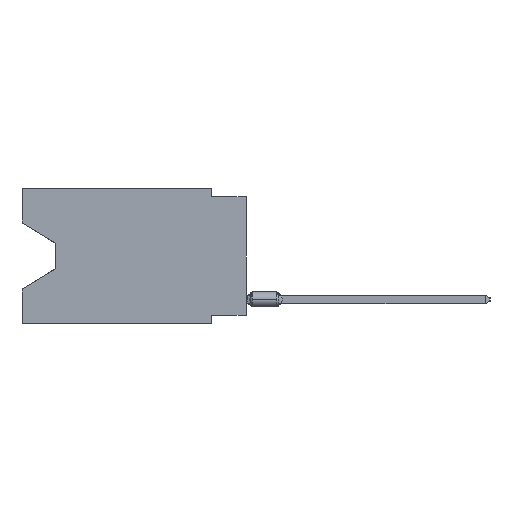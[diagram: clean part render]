
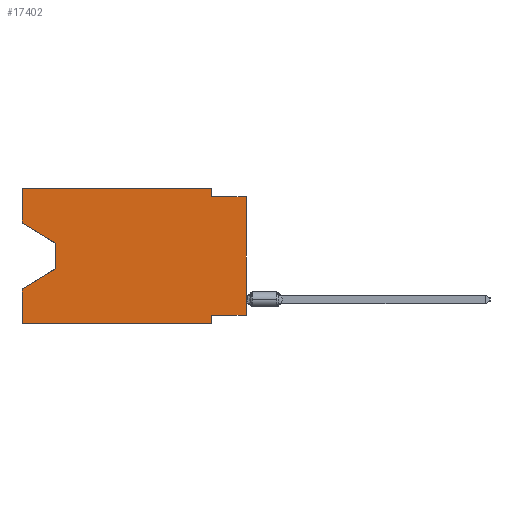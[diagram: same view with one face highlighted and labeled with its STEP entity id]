
A CAD part, left-side view. The second image highlights one B-rep face of the part: STEP entity #17402.
In plain terms, the highlighted planar face has unit normal (-1, 0, 0).
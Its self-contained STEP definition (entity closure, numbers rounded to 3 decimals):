
#490 = ORIENTED_EDGE ( 'NONE', *, *, #6611, .F. ) ;
#867 = EDGE_CURVE ( 'NONE', #46629, #14320, #31707, .T. ) ;
#884 = LINE ( 'NONE', #30411, #24680 ) ;
#920 = EDGE_CURVE ( 'NONE', #15908, #10579, #16933, .T. ) ;
#1246 = LINE ( 'NONE', #15779, #7198 ) ;
#1443 = PLANE ( 'NONE',  #12343 ) ;
#2384 = VECTOR ( 'NONE', #34736, 1000. ) ;
#2610 = ORIENTED_EDGE ( 'NONE', *, *, #28132, .T. ) ;
#2934 = VERTEX_POINT ( 'NONE', #3362 ) ;
#3362 = CARTESIAN_POINT ( 'NONE',  ( 0., 13.97, -5.893 ) ) ;
#3417 = VERTEX_POINT ( 'NONE', #43603 ) ;
#4393 = VERTEX_POINT ( 'NONE', #26133 ) ;
#4486 = VERTEX_POINT ( 'NONE', #42276 ) ;
#5261 = DIRECTION ( 'NONE',  ( 0., -1., 0. ) ) ;
#6031 = CARTESIAN_POINT ( 'NONE',  ( 0., 13.97, -5.893 ) ) ;
#6139 = CARTESIAN_POINT ( 'NONE',  ( 0., 16.383, 0. ) ) ;
#6611 = EDGE_CURVE ( 'NONE', #37154, #45701, #17321, .T. ) ;
#6680 = VECTOR ( 'NONE', #11840, 1000. ) ;
#6892 = ORIENTED_EDGE ( 'NONE', *, *, #28656, .F. ) ;
#7198 = VECTOR ( 'NONE', #44785, 1000. ) ;
#7208 = ORIENTED_EDGE ( 'NONE', *, *, #8430, .T. ) ;
#8305 = CARTESIAN_POINT ( 'NONE',  ( 0., 16.383, -9.906 ) ) ;
#8385 = ORIENTED_EDGE ( 'NONE', *, *, #867, .T. ) ;
#8430 = EDGE_CURVE ( 'NONE', #14320, #2934, #13546, .T. ) ;
#9372 = EDGE_CURVE ( 'NONE', #3417, #26324, #43079, .T. ) ;
#10579 = VERTEX_POINT ( 'NONE', #18112 ) ;
#10621 = VECTOR ( 'NONE', #16477, 1000. ) ;
#11178 = DIRECTION ( 'NONE',  ( 0., -1., 0. ) ) ;
#11235 = EDGE_CURVE ( 'NONE', #26324, #4393, #38291, .T. ) ;
#11840 = DIRECTION ( 'NONE',  ( 0., 0., -1. ) ) ;
#12310 = DIRECTION ( 'NONE',  ( 0., 0., 1. ) ) ;
#12343 = AXIS2_PLACEMENT_3D ( 'NONE', #15499, #12640, #41662 ) ;
#12640 = DIRECTION ( 'NONE',  ( 1., 0., 0. ) ) ;
#12672 = CARTESIAN_POINT ( 'NONE',  ( 0., 16.383, 0. ) ) ;
#12894 = VECTOR ( 'NONE', #20752, 1000. ) ;
#13381 = CARTESIAN_POINT ( 'NONE',  ( 0., 0., -0.635 ) ) ;
#13546 = LINE ( 'NONE', #28068, #6680 ) ;
#14320 = VERTEX_POINT ( 'NONE', #46619 ) ;
#15499 = CARTESIAN_POINT ( 'NONE',  ( 0., 16.383, 0. ) ) ;
#15779 = CARTESIAN_POINT ( 'NONE',  ( 0., 2.54, 0. ) ) ;
#15908 = VERTEX_POINT ( 'NONE', #35301 ) ;
#16450 = VECTOR ( 'NONE', #11178, 1000. ) ;
#16477 = DIRECTION ( 'NONE',  ( 0., 0., 1. ) ) ;
#16847 = ORIENTED_EDGE ( 'NONE', *, *, #9372, .F. ) ;
#16933 = LINE ( 'NONE', #13381, #36762 ) ;
#17321 = LINE ( 'NONE', #6139, #44432 ) ;
#17402 = ADVANCED_FACE ( 'NONE', ( #44979 ), #1443, .F. ) ;
#17589 = ORIENTED_EDGE ( 'NONE', *, *, #33827, .F. ) ;
#17632 = CARTESIAN_POINT ( 'NONE',  ( 0., 0., -9.271 ) ) ;
#18037 = VECTOR ( 'NONE', #38646, 1000. ) ;
#18112 = CARTESIAN_POINT ( 'NONE',  ( 0., 0., -0.635 ) ) ;
#18718 = CARTESIAN_POINT ( 'NONE',  ( 0., 2.54, -9.271 ) ) ;
#18853 = ORIENTED_EDGE ( 'NONE', *, *, #920, .F. ) ;
#19811 = ORIENTED_EDGE ( 'NONE', *, *, #11235, .F. ) ;
#20097 = CARTESIAN_POINT ( 'NONE',  ( 0., 16.383, -9.906 ) ) ;
#20220 = CARTESIAN_POINT ( 'NONE',  ( 0., 2.54, -9.906 ) ) ;
#20752 = DIRECTION ( 'NONE',  ( 0., 1., 0. ) ) ;
#20771 = DIRECTION ( 'NONE',  ( 0., -1., 0. ) ) ;
#21290 = ORIENTED_EDGE ( 'NONE', *, *, #41741, .F. ) ;
#21333 = ORIENTED_EDGE ( 'NONE', *, *, #46940, .T. ) ;
#22332 = CARTESIAN_POINT ( 'NONE',  ( 0., 16.383, -7.36 ) ) ;
#24467 = DIRECTION ( 'NONE',  ( 0., 0., 1. ) ) ;
#24680 = VECTOR ( 'NONE', #12310, 1000. ) ;
#26133 = CARTESIAN_POINT ( 'NONE',  ( 0., 2.54, -9.906 ) ) ;
#26244 = CARTESIAN_POINT ( 'NONE',  ( 0., 16.383, 0. ) ) ;
#26324 = VERTEX_POINT ( 'NONE', #18718 ) ;
#26868 = VECTOR ( 'NONE', #46414, 1000. ) ;
#27174 = CARTESIAN_POINT ( 'NONE',  ( 0., 16.383, 0. ) ) ;
#28068 = CARTESIAN_POINT ( 'NONE',  ( 0., 13.97, -4.013 ) ) ;
#28132 = EDGE_CURVE ( 'NONE', #2934, #45701, #41958, .T. ) ;
#28545 = CARTESIAN_POINT ( 'NONE',  ( 0., 16.383, -2.546 ) ) ;
#28656 = EDGE_CURVE ( 'NONE', #37343, #4486, #44768, .T. ) ;
#30411 = CARTESIAN_POINT ( 'NONE',  ( 0., 0., 0. ) ) ;
#31321 = ORIENTED_EDGE ( 'NONE', *, *, #37578, .T. ) ;
#31471 = CARTESIAN_POINT ( 'NONE',  ( 0., 16.383, -2.546 ) ) ;
#31707 = LINE ( 'NONE', #31471, #26868 ) ;
#31980 = EDGE_LOOP ( 'NONE', ( #8385, #7208, #2610, #490, #31321, #19811, #16847, #21333, #18853, #17589, #6892, #21290 ) ) ;
#33827 = EDGE_CURVE ( 'NONE', #4486, #15908, #1246, .T. ) ;
#34736 = DIRECTION ( 'NONE',  ( 0., 0., -1. ) ) ;
#35040 = LINE ( 'NONE', #12672, #10621 ) ;
#35301 = CARTESIAN_POINT ( 'NONE',  ( 0., 2.54, -0.635 ) ) ;
#35574 = VECTOR ( 'NONE', #5261, 1000. ) ;
#36762 = VECTOR ( 'NONE', #20771, 1000. ) ;
#37154 = VERTEX_POINT ( 'NONE', #20097 ) ;
#37343 = VERTEX_POINT ( 'NONE', #26244 ) ;
#37578 = EDGE_CURVE ( 'NONE', #37154, #4393, #43763, .T. ) ;
#38291 = LINE ( 'NONE', #20220, #2384 ) ;
#38646 = DIRECTION ( 'NONE',  ( 0., 0.855, -0.519 ) ) ;
#41662 = DIRECTION ( 'NONE',  ( 0., 0., -1. ) ) ;
#41741 = EDGE_CURVE ( 'NONE', #46629, #37343, #35040, .T. ) ;
#41958 = LINE ( 'NONE', #6031, #18037 ) ;
#42276 = CARTESIAN_POINT ( 'NONE',  ( 0., 2.54, 0. ) ) ;
#43079 = LINE ( 'NONE', #17632, #12894 ) ;
#43603 = CARTESIAN_POINT ( 'NONE',  ( 0., 0., -9.271 ) ) ;
#43763 = LINE ( 'NONE', #8305, #16450 ) ;
#44432 = VECTOR ( 'NONE', #24467, 1000. ) ;
#44768 = LINE ( 'NONE', #27174, #35574 ) ;
#44785 = DIRECTION ( 'NONE',  ( 0., 0., -1. ) ) ;
#44979 = FACE_OUTER_BOUND ( 'NONE', #31980, .T. ) ;
#45701 = VERTEX_POINT ( 'NONE', #22332 ) ;
#46414 = DIRECTION ( 'NONE',  ( 0., -0.855, -0.519 ) ) ;
#46619 = CARTESIAN_POINT ( 'NONE',  ( 0., 13.97, -4.013 ) ) ;
#46629 = VERTEX_POINT ( 'NONE', #28545 ) ;
#46940 = EDGE_CURVE ( 'NONE', #3417, #10579, #884, .T. ) ;
